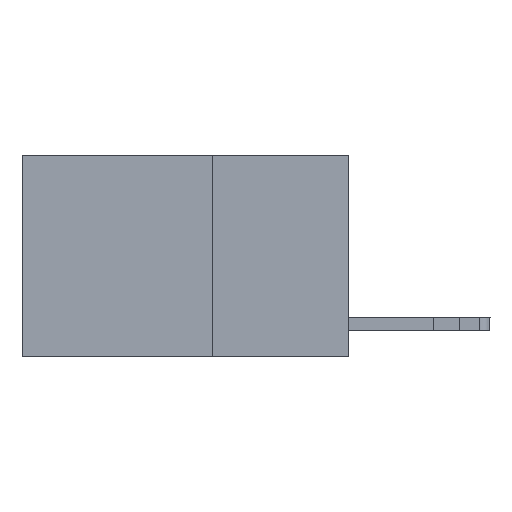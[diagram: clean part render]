
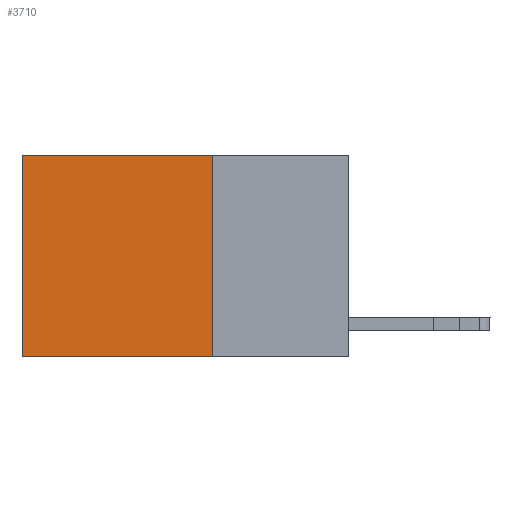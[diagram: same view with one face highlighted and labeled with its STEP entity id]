
A CAD part, left-side view. The second image highlights one B-rep face of the part: STEP entity #3710.
In plain terms, the highlighted planar face has unit normal (-1, 0, 0).
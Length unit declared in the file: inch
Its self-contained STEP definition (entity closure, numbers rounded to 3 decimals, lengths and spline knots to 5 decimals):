
#388 = LINE ( 'NONE', #2421, #19338 ) ;
#507 = VERTEX_POINT ( 'NONE', #19694 ) ;
#1825 = VECTOR ( 'NONE', #22391, 39.37008 ) ;
#2328 = AXIS2_PLACEMENT_3D ( 'NONE', #14430, #18107, #7149 ) ;
#2421 = CARTESIAN_POINT ( 'NONE',  ( 0.2625, 0.25, -0.37 ) ) ;
#3059 = DIRECTION ( 'NONE',  ( 0., 1., 0. ) ) ;
#3254 = DIRECTION ( 'NONE',  ( 0., 0., -1. ) ) ;
#3710 = ADVANCED_FACE ( 'NONE', ( #20394 ), #19883, .F. ) ;
#4038 = CARTESIAN_POINT ( 'NONE',  ( 0.2625, 0.6, 0. ) ) ;
#4592 = CARTESIAN_POINT ( 'NONE',  ( 0.2625, 0.6, 0. ) ) ;
#4851 = EDGE_CURVE ( 'NONE', #23022, #10476, #11569, .T. ) ;
#6817 = ORIENTED_EDGE ( 'NONE', *, *, #19561, .F. ) ;
#7149 = DIRECTION ( 'NONE',  ( 0., 0., -1. ) ) ;
#9074 = VECTOR ( 'NONE', #3254, 39.37008 ) ;
#10346 = CARTESIAN_POINT ( 'NONE',  ( 0.2625, 0.25, 0. ) ) ;
#10476 = VERTEX_POINT ( 'NONE', #19754 ) ;
#11355 = VECTOR ( 'NONE', #3059, 39.37008 ) ;
#11569 = LINE ( 'NONE', #4038, #1825 ) ;
#11781 = VERTEX_POINT ( 'NONE', #21806 ) ;
#14430 = CARTESIAN_POINT ( 'NONE',  ( 0.2625, 0.25, 0. ) ) ;
#14511 = LINE ( 'NONE', #23467, #9074 ) ;
#18107 = DIRECTION ( 'NONE',  ( 1., 0., 0. ) ) ;
#18932 = DIRECTION ( 'NONE',  ( 0., 1., 0. ) ) ;
#19172 = ORIENTED_EDGE ( 'NONE', *, *, #20420, .F. ) ;
#19338 = VECTOR ( 'NONE', #18932, 39.37008 ) ;
#19561 = EDGE_CURVE ( 'NONE', #507, #11781, #14511, .T. ) ;
#19694 = CARTESIAN_POINT ( 'NONE',  ( 0.2625, 0.25, 0. ) ) ;
#19698 = ORIENTED_EDGE ( 'NONE', *, *, #4851, .T. ) ;
#19754 = CARTESIAN_POINT ( 'NONE',  ( 0.2625, 0.6, -0.37 ) ) ;
#19883 = PLANE ( 'NONE',  #2328 ) ;
#20073 = EDGE_LOOP ( 'NONE', ( #19698, #19172, #6817, #20176 ) ) ;
#20176 = ORIENTED_EDGE ( 'NONE', *, *, #23117, .T. ) ;
#20394 = FACE_OUTER_BOUND ( 'NONE', #20073, .T. ) ;
#20420 = EDGE_CURVE ( 'NONE', #11781, #10476, #388, .T. ) ;
#20576 = LINE ( 'NONE', #10346, #11355 ) ;
#21806 = CARTESIAN_POINT ( 'NONE',  ( 0.2625, 0.25, -0.37 ) ) ;
#22391 = DIRECTION ( 'NONE',  ( 0., 0., -1. ) ) ;
#23022 = VERTEX_POINT ( 'NONE', #4592 ) ;
#23117 = EDGE_CURVE ( 'NONE', #507, #23022, #20576, .T. ) ;
#23467 = CARTESIAN_POINT ( 'NONE',  ( 0.2625, 0.25, 0. ) ) ;
